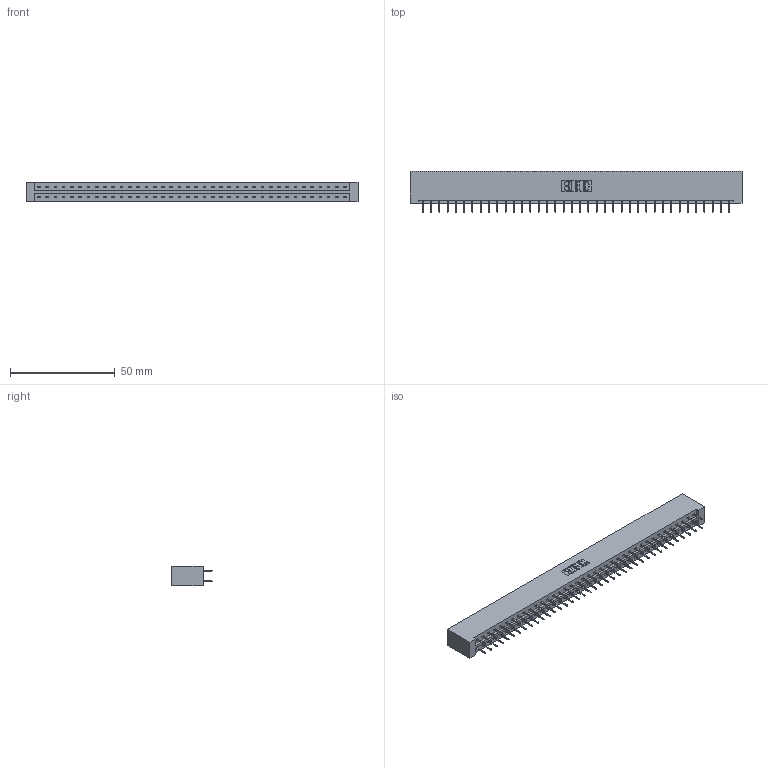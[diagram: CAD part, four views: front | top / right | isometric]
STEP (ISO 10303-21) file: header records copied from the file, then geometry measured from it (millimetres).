
FILE_DESCRIPTION (( 'STEP AP203' ), '1' );
FILE_NAME ('833-076-524-201.STEP', '2020-06-05T18:09:10', ( '' ), ( '' ), 'SwSTEP 2.0', 'SolidWorks 2020', '' );
FILE_SCHEMA (( 'CONFIG_CONTROL_DESIGN' ));
Length unit declared in the file: inch
Products named in the file (3): 345-292-001_345-293-124; 833-076-524-201; 833 Part_Lugless
Assembly tree (77 placements, depth 2):
  833-076-524-201
    833 Part_Lugless
    345-292-001_345-293-124  x76
Bounding box: 158.83 x 19.69 x 9.4 mm (x, y, z)
Volume: 16695.1 mm3; surface area: 19373.9 mm2
Topology: 77 solids, 77 shells, 4362 faces, 12371 edges, 7942 vertices
Faces by surface type: plane 3258, cylinder 1104
Entity records: 24761 total; most frequent: CARTESIAN_POINT 4106, ORIENTED_EDGE 4042, DIRECTION 3509, EDGE_CURVE 2021, VECTOR 1905, LINE 1905, VERTEX_POINT 1342, AXIS2_PLACEMENT_3D 802
